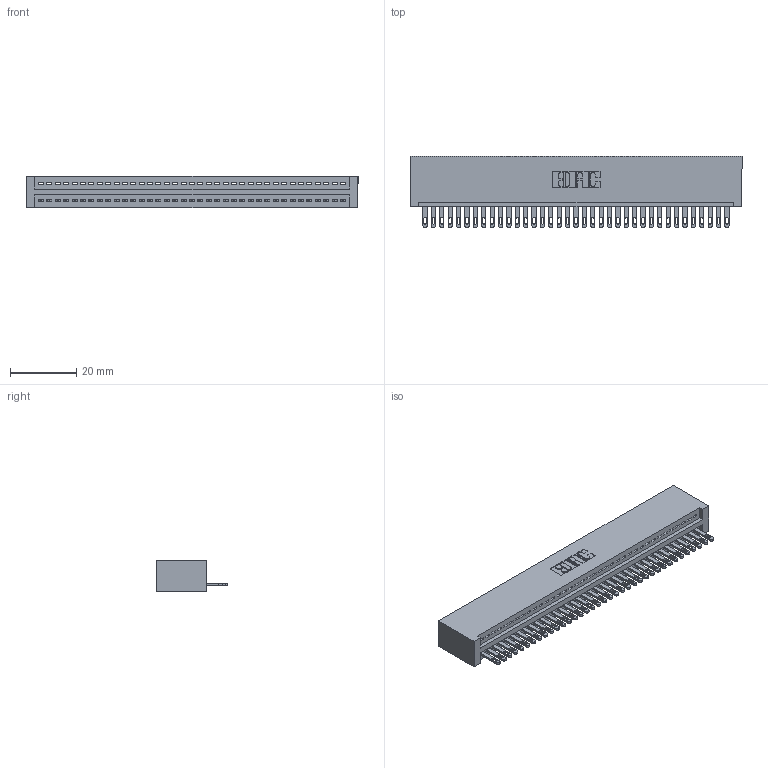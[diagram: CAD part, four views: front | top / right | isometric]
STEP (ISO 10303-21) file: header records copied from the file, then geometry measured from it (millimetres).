
FILE_DESCRIPTION (( 'STEP AP203' ), '1' );
FILE_NAME ('345-037-500-101.STEP', '2019-10-08T00:09:45', ( '' ), ( '' ), 'SwSTEP 2.0', 'SolidWorks 2016', '' );
FILE_SCHEMA (( 'CONFIG_CONTROL_DESIGN' ));
Length unit declared in the file: inch
Products named in the file (3): 345-292-001_345-293-100; 345-037-500-101; 345 Part_No Mounting Lugs
Assembly tree (38 placements, depth 2):
  345-037-500-101
    345 Part_No Mounting Lugs
    345-292-001_345-293-100  x37
Bounding box: 100.58 x 21.51 x 9.4 mm (x, y, z)
Volume: 10119.9 mm3; surface area: 13653.7 mm2
Topology: 38 solids, 38 shells, 2116 faces, 6533 edges, 4354 vertices
Faces by surface type: plane 1334, cylinder 782
Entity records: 28173 total; most frequent: CARTESIAN_POINT 4887, ORIENTED_EDGE 4858, DIRECTION 4271, EDGE_CURVE 2429, VECTOR 2153, LINE 2153, VERTEX_POINT 1618, AXIS2_PLACEMENT_3D 1059
